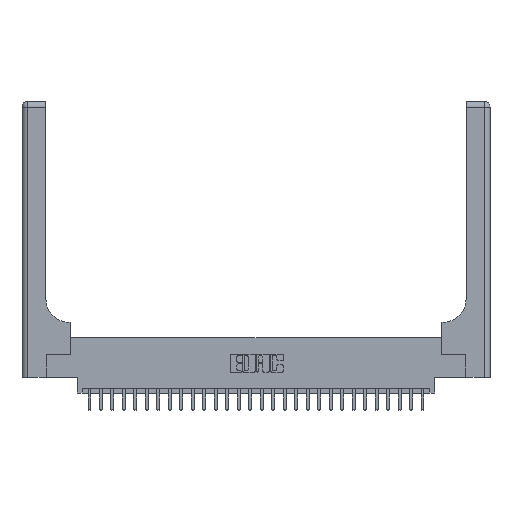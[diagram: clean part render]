
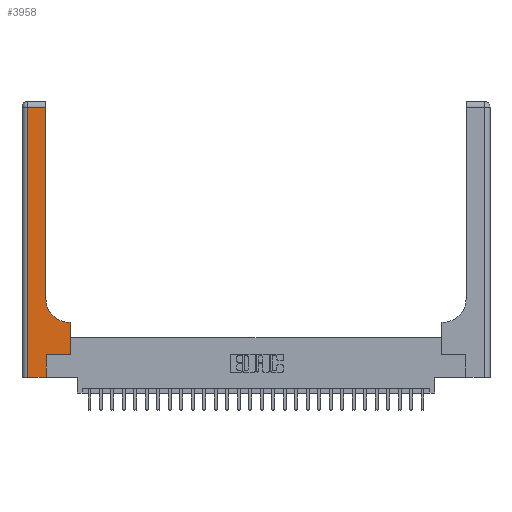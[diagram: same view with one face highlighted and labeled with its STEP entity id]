
A CAD part, top view. The second image highlights one B-rep face of the part: STEP entity #3958.
In plain terms, the highlighted planar face has unit normal (0, 0, 1).
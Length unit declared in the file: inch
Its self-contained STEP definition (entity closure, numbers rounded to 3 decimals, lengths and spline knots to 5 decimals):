
#54 = LINE ( 'NONE', #1987, #26022 ) ;
#156 = EDGE_CURVE ( 'NONE', #4991, #16452, #1165, .T. ) ;
#186 = VECTOR ( 'NONE', #15722, 39.37008 ) ;
#258 = EDGE_CURVE ( 'NONE', #26616, #2682, #54, .T. ) ;
#575 = ORIENTED_EDGE ( 'NONE', *, *, #12025, .T. ) ;
#1165 = LINE ( 'NONE', #18472, #26880 ) ;
#1451 = EDGE_CURVE ( 'NONE', #2682, #23572, #7305, .T. ) ;
#1523 = CARTESIAN_POINT ( 'NONE',  ( 0.26, 3., 0.37 ) ) ;
#1572 = DIRECTION ( 'NONE',  ( 0., 1., 0. ) ) ;
#1865 = DIRECTION ( 'NONE',  ( 1., 0., 0. ) ) ;
#1987 = CARTESIAN_POINT ( 'NONE',  ( 0., 2.94, 0.37 ) ) ;
#2212 = VECTOR ( 'NONE', #6895, 39.37008 ) ;
#2506 = LINE ( 'NONE', #25799, #186 ) ;
#2682 = VERTEX_POINT ( 'NONE', #3445 ) ;
#3445 = CARTESIAN_POINT ( 'NONE',  ( 0.06, 2.94, 0.37 ) ) ;
#3662 = ORIENTED_EDGE ( 'NONE', *, *, #23817, .T. ) ;
#3697 = EDGE_CURVE ( 'NONE', #16742, #18353, #20905, .T. ) ;
#3888 = ORIENTED_EDGE ( 'NONE', *, *, #156, .T. ) ;
#3898 = LINE ( 'NONE', #12322, #21579 ) ;
#3958 = ADVANCED_FACE ( 'NONE', ( #6332 ), #8762, .F. ) ;
#4508 = CARTESIAN_POINT ( 'NONE',  ( 0.528, 0.25, 0.37 ) ) ;
#4991 = VERTEX_POINT ( 'NONE', #15181 ) ;
#5495 = EDGE_LOOP ( 'NONE', ( #11137, #5948, #7912, #13276, #3888, #575, #20713, #3662, #14059 ) ) ;
#5862 = CARTESIAN_POINT ( 'NONE',  ( 0.26, 2.94, 0.37 ) ) ;
#5948 = ORIENTED_EDGE ( 'NONE', *, *, #258, .T. ) ;
#6332 = FACE_OUTER_BOUND ( 'NONE', #5495, .T. ) ;
#6488 = CARTESIAN_POINT ( 'NONE',  ( 0.528, 0.6, 0.37 ) ) ;
#6895 = DIRECTION ( 'NONE',  ( 1., 0., 0. ) ) ;
#7305 = LINE ( 'NONE', #9323, #7687 ) ;
#7539 = LINE ( 'NONE', #1523, #13086 ) ;
#7687 = VECTOR ( 'NONE', #23897, 39.37008 ) ;
#7798 = EDGE_CURVE ( 'NONE', #23572, #4991, #3898, .T. ) ;
#7912 = ORIENTED_EDGE ( 'NONE', *, *, #1451, .T. ) ;
#8607 = AXIS2_PLACEMENT_3D ( 'NONE', #8919, #19922, #11037 ) ;
#8762 = PLANE ( 'NONE',  #26269 ) ;
#8848 = VERTEX_POINT ( 'NONE', #4508 ) ;
#8919 = CARTESIAN_POINT ( 'NONE',  ( 0.51, 0.85, 0.37 ) ) ;
#9323 = CARTESIAN_POINT ( 'NONE',  ( 0.06, 3., 0.37 ) ) ;
#10144 = DIRECTION ( 'NONE',  ( 0., 1., 0. ) ) ;
#11037 = DIRECTION ( 'NONE',  ( 1., 0., 0. ) ) ;
#11137 = ORIENTED_EDGE ( 'NONE', *, *, #25610, .T. ) ;
#12025 = EDGE_CURVE ( 'NONE', #16452, #8848, #17342, .T. ) ;
#12322 = CARTESIAN_POINT ( 'NONE',  ( 0., 0., 0.37 ) ) ;
#12937 = VECTOR ( 'NONE', #10144, 39.37008 ) ;
#13086 = VECTOR ( 'NONE', #14168, 39.37008 ) ;
#13276 = ORIENTED_EDGE ( 'NONE', *, *, #7798, .T. ) ;
#14059 = ORIENTED_EDGE ( 'NONE', *, *, #3697, .T. ) ;
#14168 = DIRECTION ( 'NONE',  ( 0., 1., 0. ) ) ;
#14443 = VERTEX_POINT ( 'NONE', #6488 ) ;
#14985 = LINE ( 'NONE', #17300, #12937 ) ;
#15181 = CARTESIAN_POINT ( 'NONE',  ( 0.265, 0., 0.37 ) ) ;
#15722 = DIRECTION ( 'NONE',  ( -1., 0., 0. ) ) ;
#16452 = VERTEX_POINT ( 'NONE', #24367 ) ;
#16742 = VERTEX_POINT ( 'NONE', #21597 ) ;
#16791 = CARTESIAN_POINT ( 'NONE',  ( 0., 3., 0.37 ) ) ;
#17300 = CARTESIAN_POINT ( 'NONE',  ( 0.528, 0.25, 0.37 ) ) ;
#17342 = LINE ( 'NONE', #25783, #2212 ) ;
#18353 = VERTEX_POINT ( 'NONE', #21655 ) ;
#18472 = CARTESIAN_POINT ( 'NONE',  ( 0.265, 0., 0.37 ) ) ;
#19922 = DIRECTION ( 'NONE',  ( 0., 0., -1. ) ) ;
#20713 = ORIENTED_EDGE ( 'NONE', *, *, #24038, .T. ) ;
#20905 = CIRCLE ( 'NONE', #8607, 0.25 ) ;
#21016 = DIRECTION ( 'NONE',  ( -1., 0., 0. ) ) ;
#21579 = VECTOR ( 'NONE', #1865, 39.37008 ) ;
#21597 = CARTESIAN_POINT ( 'NONE',  ( 0.51, 0.6, 0.37 ) ) ;
#21655 = CARTESIAN_POINT ( 'NONE',  ( 0.26, 0.85, 0.37 ) ) ;
#23077 = DIRECTION ( 'NONE',  ( -1., 0., 0. ) ) ;
#23193 = DIRECTION ( 'NONE',  ( 0., 0., -1. ) ) ;
#23572 = VERTEX_POINT ( 'NONE', #25393 ) ;
#23817 = EDGE_CURVE ( 'NONE', #14443, #16742, #2506, .T. ) ;
#23897 = DIRECTION ( 'NONE',  ( 0., -1., 0. ) ) ;
#24038 = EDGE_CURVE ( 'NONE', #8848, #14443, #14985, .T. ) ;
#24367 = CARTESIAN_POINT ( 'NONE',  ( 0.265, 0.25, 0.37 ) ) ;
#25393 = CARTESIAN_POINT ( 'NONE',  ( 0.06, 0., 0.37 ) ) ;
#25610 = EDGE_CURVE ( 'NONE', #18353, #26616, #7539, .T. ) ;
#25783 = CARTESIAN_POINT ( 'NONE',  ( 0.265, 0.25, 0.37 ) ) ;
#25799 = CARTESIAN_POINT ( 'NONE',  ( 0.26, 0.6, 0.37 ) ) ;
#26022 = VECTOR ( 'NONE', #23077, 39.37008 ) ;
#26269 = AXIS2_PLACEMENT_3D ( 'NONE', #16791, #23193, #21016 ) ;
#26616 = VERTEX_POINT ( 'NONE', #5862 ) ;
#26880 = VECTOR ( 'NONE', #1572, 39.37008 ) ;
